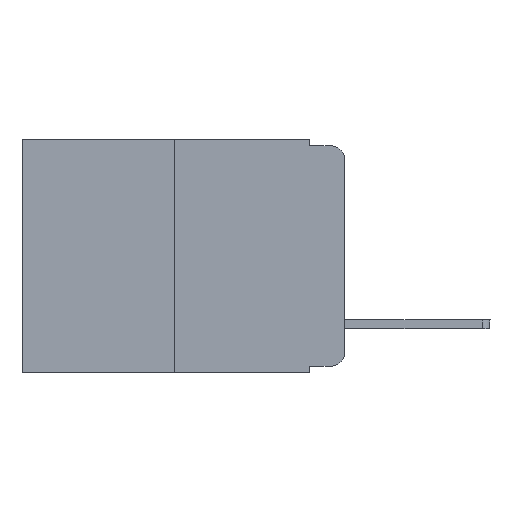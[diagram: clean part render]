
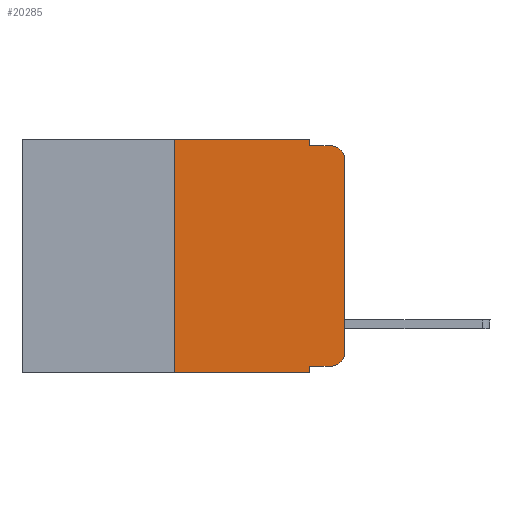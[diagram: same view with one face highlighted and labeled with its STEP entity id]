
A CAD part, left-side view. The second image highlights one B-rep face of the part: STEP entity #20285.
In plain terms, the highlighted planar face has unit normal (-1, 0, 0).
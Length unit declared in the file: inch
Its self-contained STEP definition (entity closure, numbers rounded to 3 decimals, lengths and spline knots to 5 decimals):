
#380 = DIRECTION ( 'NONE',  ( 0., 0., -1. ) ) ;
#452 = DIRECTION ( 'NONE',  ( 0., 0., -1. ) ) ;
#741 = VERTEX_POINT ( 'NONE', #21735 ) ;
#814 = VECTOR ( 'NONE', #10086, 39.37008 ) ;
#944 = LINE ( 'NONE', #12205, #814 ) ;
#1066 = CARTESIAN_POINT ( 'NONE',  ( 0., 0., -0.03 ) ) ;
#1232 = CARTESIAN_POINT ( 'NONE',  ( 0., 0.25, -0.343 ) ) ;
#1390 = VERTEX_POINT ( 'NONE', #23435 ) ;
#1427 = VERTEX_POINT ( 'NONE', #1066 ) ;
#1756 = DIRECTION ( 'NONE',  ( -1., 0., 0. ) ) ;
#1791 = VERTEX_POINT ( 'NONE', #9928 ) ;
#2583 = CARTESIAN_POINT ( 'NONE',  ( 0., 0.25, 0. ) ) ;
#2599 = VECTOR ( 'NONE', #8311, 39.37008 ) ;
#2839 = CARTESIAN_POINT ( 'NONE',  ( 0., 0.051, -0.01 ) ) ;
#3783 = ORIENTED_EDGE ( 'NONE', *, *, #15319, .T. ) ;
#3791 = EDGE_CURVE ( 'NONE', #1427, #9689, #4501, .T. ) ;
#3853 = LINE ( 'NONE', #22797, #19139 ) ;
#4486 = VECTOR ( 'NONE', #20215, 39.37008 ) ;
#4501 = CIRCLE ( 'NONE', #15671, 0.02 ) ;
#4614 = LINE ( 'NONE', #2839, #5328 ) ;
#5237 = CARTESIAN_POINT ( 'NONE',  ( 0., 0., 0. ) ) ;
#5328 = VECTOR ( 'NONE', #18672, 39.37008 ) ;
#5355 = VECTOR ( 'NONE', #20339, 39.37008 ) ;
#6807 = VERTEX_POINT ( 'NONE', #18639 ) ;
#7224 = DIRECTION ( 'NONE',  ( 1., 0., 0. ) ) ;
#7509 = VERTEX_POINT ( 'NONE', #16089 ) ;
#7633 = ORIENTED_EDGE ( 'NONE', *, *, #17985, .F. ) ;
#7686 = EDGE_CURVE ( 'NONE', #17388, #1390, #3853, .T. ) ;
#8221 = VERTEX_POINT ( 'NONE', #1232 ) ;
#8303 = ORIENTED_EDGE ( 'NONE', *, *, #21993, .T. ) ;
#8311 = DIRECTION ( 'NONE',  ( 0., 0., 1. ) ) ;
#8928 = DIRECTION ( 'NONE',  ( -1., 0., 0. ) ) ;
#9371 = CARTESIAN_POINT ( 'NONE',  ( 0., 0.02, -0.03 ) ) ;
#9487 = PLANE ( 'NONE',  #19764 ) ;
#9689 = VERTEX_POINT ( 'NONE', #9930 ) ;
#9928 = CARTESIAN_POINT ( 'NONE',  ( 0., 0.051, 0. ) ) ;
#9930 = CARTESIAN_POINT ( 'NONE',  ( 0., 0.02, -0.01 ) ) ;
#10086 = DIRECTION ( 'NONE',  ( 0., -1., 0. ) ) ;
#10354 = ORIENTED_EDGE ( 'NONE', *, *, #19793, .F. ) ;
#11209 = AXIS2_PLACEMENT_3D ( 'NONE', #12435, #8928, #20295 ) ;
#11932 = DIRECTION ( 'NONE',  ( 0., -1., 0. ) ) ;
#12205 = CARTESIAN_POINT ( 'NONE',  ( 0., 0.473, -0.343 ) ) ;
#12435 = CARTESIAN_POINT ( 'NONE',  ( 0., 0.02, -0.313 ) ) ;
#12576 = EDGE_CURVE ( 'NONE', #1791, #741, #19288, .T. ) ;
#12605 = LINE ( 'NONE', #5237, #4486 ) ;
#12728 = CARTESIAN_POINT ( 'NONE',  ( 0., 0.473, 0. ) ) ;
#13242 = VERTEX_POINT ( 'NONE', #24271 ) ;
#15319 = EDGE_CURVE ( 'NONE', #7509, #1427, #12605, .T. ) ;
#15387 = CARTESIAN_POINT ( 'NONE',  ( 0., 0.051, -0.333 ) ) ;
#15671 = AXIS2_PLACEMENT_3D ( 'NONE', #9371, #1756, #380 ) ;
#16039 = VECTOR ( 'NONE', #11932, 39.37008 ) ;
#16088 = ORIENTED_EDGE ( 'NONE', *, *, #23589, .T. ) ;
#16089 = CARTESIAN_POINT ( 'NONE',  ( 0., 0., -0.313 ) ) ;
#16991 = CARTESIAN_POINT ( 'NONE',  ( 0., 0.473, 0. ) ) ;
#17109 = DIRECTION ( 'NONE',  ( 0., 0., -1. ) ) ;
#17290 = DIRECTION ( 'NONE',  ( 0., 0., -1. ) ) ;
#17388 = VERTEX_POINT ( 'NONE', #15387 ) ;
#17420 = CARTESIAN_POINT ( 'NONE',  ( 0., 0.051, 0. ) ) ;
#17435 = ORIENTED_EDGE ( 'NONE', *, *, #3791, .T. ) ;
#17501 = ORIENTED_EDGE ( 'NONE', *, *, #23085, .T. ) ;
#17985 = EDGE_CURVE ( 'NONE', #741, #9689, #4614, .T. ) ;
#18410 = EDGE_LOOP ( 'NONE', ( #3783, #17435, #7633, #22886, #22080, #10354, #17501, #21313, #16088, #8303 ) ) ;
#18639 = CARTESIAN_POINT ( 'NONE',  ( 0., 0.25, 0. ) ) ;
#18672 = DIRECTION ( 'NONE',  ( 0., -1., 0. ) ) ;
#18899 = EDGE_CURVE ( 'NONE', #6807, #1791, #22201, .T. ) ;
#19139 = VECTOR ( 'NONE', #452, 39.37008 ) ;
#19288 = LINE ( 'NONE', #17420, #22283 ) ;
#19764 = AXIS2_PLACEMENT_3D ( 'NONE', #16991, #7224, #17109 ) ;
#19793 = EDGE_CURVE ( 'NONE', #8221, #6807, #21895, .T. ) ;
#19910 = CARTESIAN_POINT ( 'NONE',  ( 0., 0.051, -0.333 ) ) ;
#20215 = DIRECTION ( 'NONE',  ( 0., 0., 1. ) ) ;
#20285 = ADVANCED_FACE ( 'NONE', ( #24341 ), #9487, .F. ) ;
#20295 = DIRECTION ( 'NONE',  ( 0., 0., -1. ) ) ;
#20339 = DIRECTION ( 'NONE',  ( 0., -1., 0. ) ) ;
#21313 = ORIENTED_EDGE ( 'NONE', *, *, #7686, .F. ) ;
#21735 = CARTESIAN_POINT ( 'NONE',  ( 0., 0.051, -0.01 ) ) ;
#21895 = LINE ( 'NONE', #2583, #2599 ) ;
#21993 = EDGE_CURVE ( 'NONE', #13242, #7509, #23171, .T. ) ;
#22080 = ORIENTED_EDGE ( 'NONE', *, *, #18899, .F. ) ;
#22201 = LINE ( 'NONE', #12728, #5355 ) ;
#22283 = VECTOR ( 'NONE', #17290, 39.37008 ) ;
#22797 = CARTESIAN_POINT ( 'NONE',  ( 0., 0.051, 0. ) ) ;
#22886 = ORIENTED_EDGE ( 'NONE', *, *, #12576, .F. ) ;
#23085 = EDGE_CURVE ( 'NONE', #8221, #1390, #944, .T. ) ;
#23171 = CIRCLE ( 'NONE', #11209, 0.02 ) ;
#23435 = CARTESIAN_POINT ( 'NONE',  ( 0., 0.051, -0.343 ) ) ;
#23589 = EDGE_CURVE ( 'NONE', #17388, #13242, #23658, .T. ) ;
#23658 = LINE ( 'NONE', #19910, #16039 ) ;
#24271 = CARTESIAN_POINT ( 'NONE',  ( 0., 0.02, -0.333 ) ) ;
#24341 = FACE_OUTER_BOUND ( 'NONE', #18410, .T. ) ;
